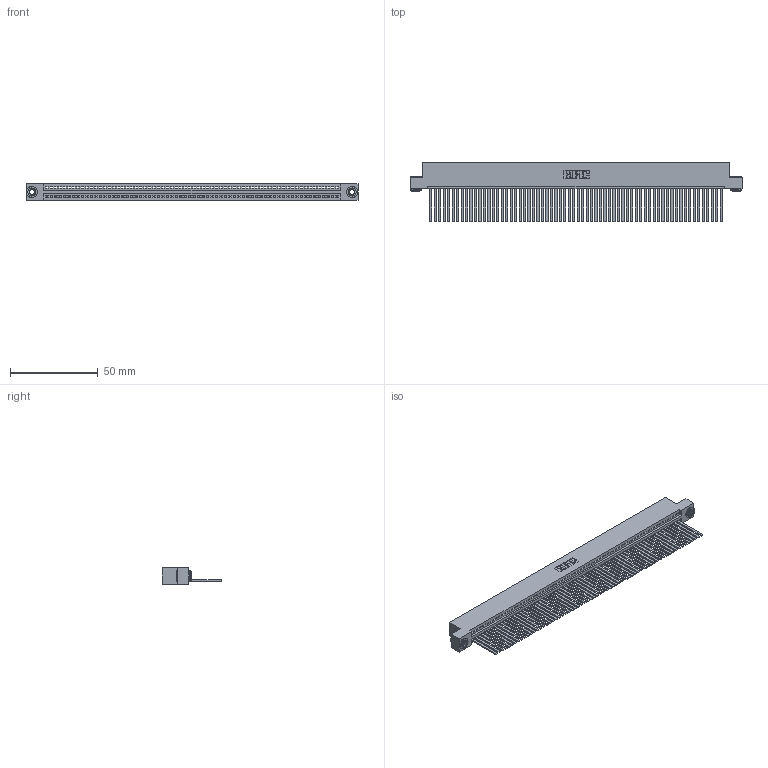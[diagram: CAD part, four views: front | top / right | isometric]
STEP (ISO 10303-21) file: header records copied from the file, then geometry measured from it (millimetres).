
FILE_DESCRIPTION (( 'STEP AP203' ), '1' );
FILE_NAME ('345-066-544-103.STEP', '2018-09-28T22:34:56', ( '' ), ( '' ), 'SwSTEP 2.0', 'SolidWorks 2016', '' );
FILE_SCHEMA (( 'CONFIG_CONTROL_DESIGN' ));
Length unit declared in the file: inch
Products named in the file (4): 345 Part_Flush Mounting Lugs - 0.156 Dia-TH; 345-250-002_345-250-002-102; 345-066-544-103; 345-292-001_345-293-144
Assembly tree (69 placements, depth 2):
  345-066-544-103
    345 Part_Flush Mounting Lugs - 0.156 Dia-TH
    345-292-001_345-293-144  x66
    345-250-002_345-250-002-102  x2
Bounding box: 188.85 x 33.96 x 9.4 mm (x, y, z)
Volume: 18917.4 mm3; surface area: 27974.9 mm2
Topology: 69 solids, 69 shells, 3596 faces, 10845 edges, 7138 vertices
Faces by surface type: plane 2466, cylinder 1122, cone 8
Entity records: 46908 total; most frequent: CARTESIAN_POINT 8101, ORIENTED_EDGE 8094, DIRECTION 7069, EDGE_CURVE 4047, LINE 3631, VECTOR 3631, VERTEX_POINT 2694, AXIS2_PLACEMENT_3D 1719
